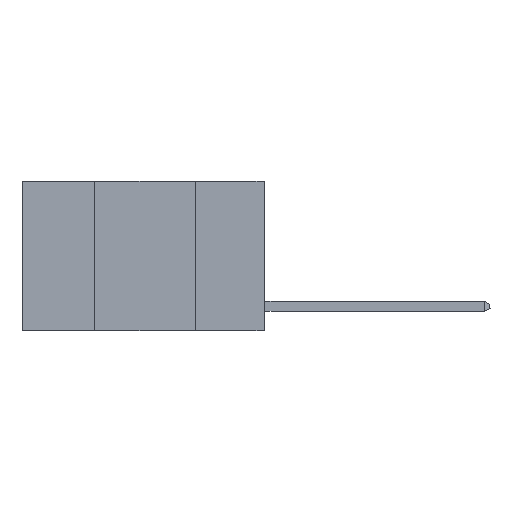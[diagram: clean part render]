
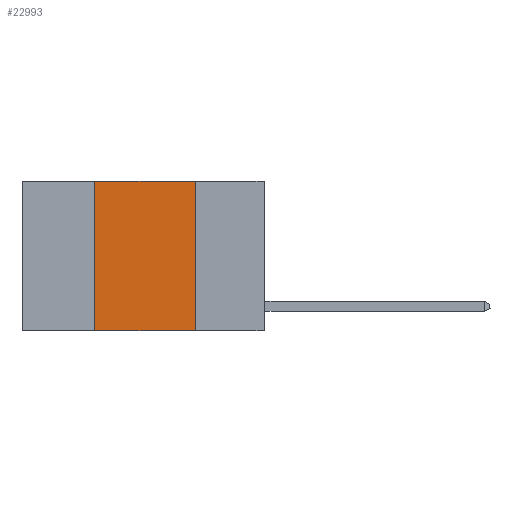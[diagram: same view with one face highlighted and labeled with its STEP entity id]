
A CAD part, left-side view. The second image highlights one B-rep face of the part: STEP entity #22993.
In plain terms, the highlighted planar face has unit normal (-1, 0, 0).
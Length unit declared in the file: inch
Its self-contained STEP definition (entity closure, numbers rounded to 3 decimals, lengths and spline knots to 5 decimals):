
#534 = ORIENTED_EDGE ( 'NONE', *, *, #6558, .T. ) ;
#858 = CARTESIAN_POINT ( 'NONE',  ( 0., 0.6, 0. ) ) ;
#1634 = VECTOR ( 'NONE', #7270, 39.37008 ) ;
#2003 = ORIENTED_EDGE ( 'NONE', *, *, #3433, .F. ) ;
#2257 = ORIENTED_EDGE ( 'NONE', *, *, #19980, .F. ) ;
#2340 = DIRECTION ( 'NONE',  ( 0., -1., 0. ) ) ;
#3433 = EDGE_CURVE ( 'NONE', #11630, #4823, #23260, .T. ) ;
#3443 = VECTOR ( 'NONE', #2340, 39.37008 ) ;
#4282 = CARTESIAN_POINT ( 'NONE',  ( 0., 0.17, 0. ) ) ;
#4823 = VERTEX_POINT ( 'NONE', #12240 ) ;
#5452 = LINE ( 'NONE', #23697, #9355 ) ;
#6510 = CARTESIAN_POINT ( 'NONE',  ( 0., 0.17, 0. ) ) ;
#6558 = EDGE_CURVE ( 'NONE', #9729, #4823, #9076, .T. ) ;
#7270 = DIRECTION ( 'NONE',  ( 0., -1., 0. ) ) ;
#9076 = LINE ( 'NONE', #16576, #1634 ) ;
#9355 = VECTOR ( 'NONE', #20163, 39.37008 ) ;
#9682 = VECTOR ( 'NONE', #23022, 39.37008 ) ;
#9729 = VERTEX_POINT ( 'NONE', #22164 ) ;
#10180 = LINE ( 'NONE', #858, #3443 ) ;
#11001 = FACE_OUTER_BOUND ( 'NONE', #19580, .T. ) ;
#11630 = VERTEX_POINT ( 'NONE', #4282 ) ;
#12120 = AXIS2_PLACEMENT_3D ( 'NONE', #23903, #18515, #22191 ) ;
#12240 = CARTESIAN_POINT ( 'NONE',  ( 0., 0.17, -0.37 ) ) ;
#14835 = ORIENTED_EDGE ( 'NONE', *, *, #17533, .F. ) ;
#16576 = CARTESIAN_POINT ( 'NONE',  ( 0., 0.6, -0.37 ) ) ;
#17533 = EDGE_CURVE ( 'NONE', #9729, #17826, #5452, .T. ) ;
#17684 = CARTESIAN_POINT ( 'NONE',  ( 0., 0.42, 0. ) ) ;
#17826 = VERTEX_POINT ( 'NONE', #17684 ) ;
#18515 = DIRECTION ( 'NONE',  ( 1., 0., 0. ) ) ;
#19580 = EDGE_LOOP ( 'NONE', ( #2003, #2257, #14835, #534 ) ) ;
#19980 = EDGE_CURVE ( 'NONE', #17826, #11630, #10180, .T. ) ;
#20163 = DIRECTION ( 'NONE',  ( 0., 0., 1. ) ) ;
#21840 = PLANE ( 'NONE',  #12120 ) ;
#22164 = CARTESIAN_POINT ( 'NONE',  ( 0., 0.42, -0.37 ) ) ;
#22191 = DIRECTION ( 'NONE',  ( 0., 0., -1. ) ) ;
#22993 = ADVANCED_FACE ( 'NONE', ( #11001 ), #21840, .F. ) ;
#23022 = DIRECTION ( 'NONE',  ( 0., 0., -1. ) ) ;
#23260 = LINE ( 'NONE', #6510, #9682 ) ;
#23697 = CARTESIAN_POINT ( 'NONE',  ( 0., 0.42, 0. ) ) ;
#23903 = CARTESIAN_POINT ( 'NONE',  ( 0., 0.6, 0. ) ) ;
